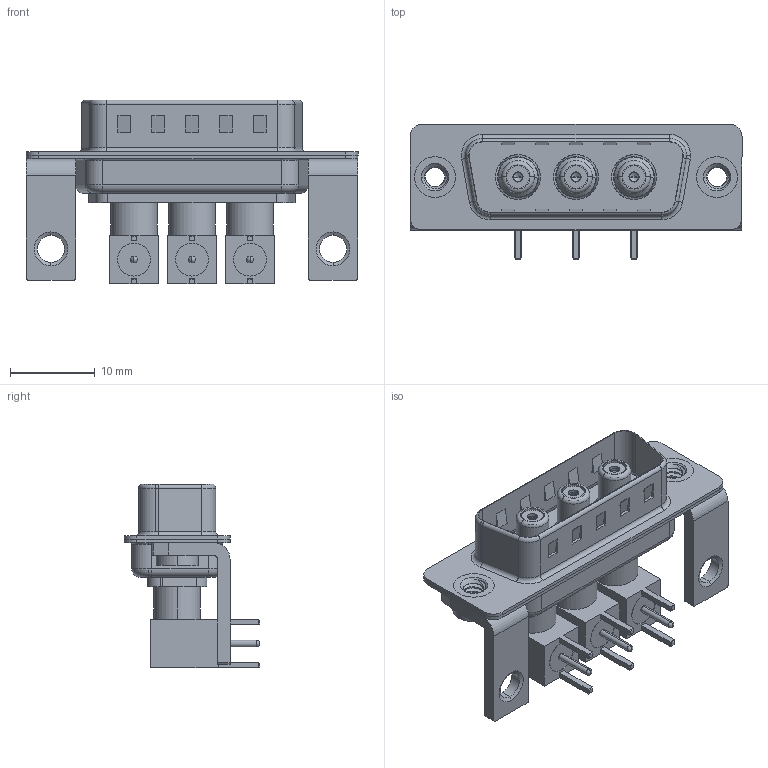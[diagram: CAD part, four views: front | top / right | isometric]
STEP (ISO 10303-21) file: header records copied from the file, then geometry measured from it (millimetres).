
FILE_DESCRIPTION (( 'STEP AP203' ), '1' );
FILE_NAME ('629-3W3-240-7TC.STEP', '2022-05-05T02:53:14', ( '' ), ( '' ), 'SwSTEP 2.0', 'SolidWorks 2020', '' );
FILE_SCHEMA (( 'CONFIG_CONTROL_DESIGN' ));
Length unit declared in the file: millimetre
Products named in the file (16): 629Combo Shell Rear_15 Contacts; 629Combo Shell Front_15 Contacts; Co-Ax Jack Assy_RA; Insulator Socket 2; Co-Ax Jack_RA PC Tail; 629Combo Housing_3W3; RA Back Shell; Socket_RA; 629Combo Stabilizer Bracket; Insulator RA Pin; Locking Collar; 629Combo Threaded Rivet_2; 629-3W3-240-7TC; Insulator Socket
Assembly tree (31 placements, depth 3):
  629-3W3-240-7TC
    629Combo Housing_3W3
    629Combo Shell Rear_15 Contacts
    629Combo Shell Front_15 Contacts
    629Combo Threaded Rivet_2  x2
    629Combo Stabilizer Bracket  x2
    Co-Ax Jack Assy_RA
      Co-Ax Jack_RA PC Tail
      Insulator Socket
      Insulator Socket 2
      Locking Collar
      Socket_RA
      RA Back Shell
      Insulator RA Pin
    Co-Ax Jack Assy_RA
      Co-Ax Jack_RA PC Tail
      Insulator Socket
      Insulator Socket 2
      Locking Collar
      Socket_RA
      RA Back Shell
      Insulator RA Pin
    Co-Ax Jack Assy_RA
      Co-Ax Jack_RA PC Tail
      Insulator Socket
      Insulator Socket 2
      Locking Collar
      Socket_RA
      RA Back Shell
      Insulator RA Pin
Bounding box: 39.2 x 16 x 21.71 mm (x, y, z)
Volume: 3008.8 mm3; surface area: 8165.2 mm2
Topology: 28 solids, 28 shells, 844 faces, 2020 edges, 1261 vertices
Faces by surface type: cylinder 358, plane 330, cone 73, torus 68, bspline 9, sphere 6
Entity records: 18341 total; most frequent: CARTESIAN_POINT 4212, DIRECTION 2668, ORIENTED_EDGE 2394, EDGE_CURVE 1197, AXIS2_PLACEMENT_3D 1010, VERTEX_POINT 755, VECTOR 648, LINE 648
